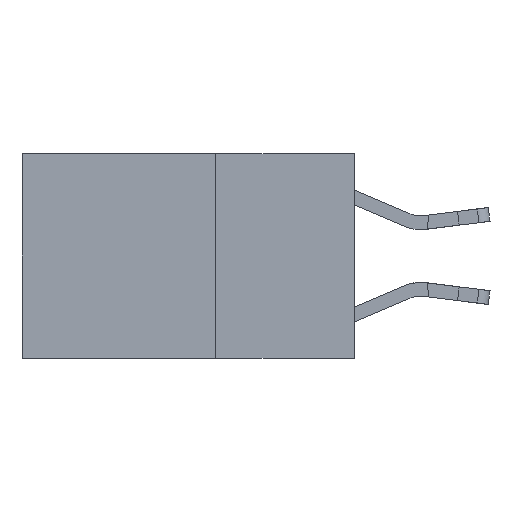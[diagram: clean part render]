
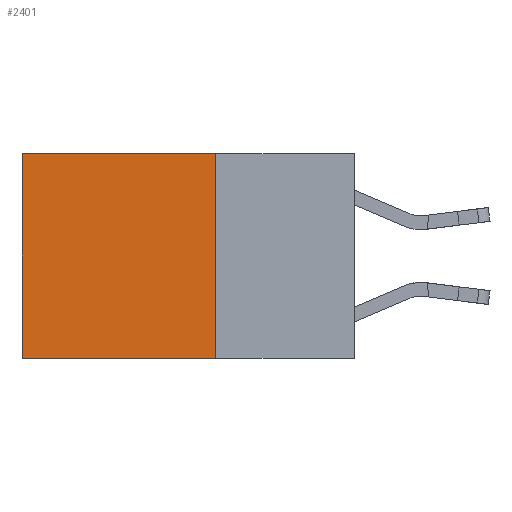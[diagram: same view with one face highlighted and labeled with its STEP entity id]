
A CAD part, left-side view. The second image highlights one B-rep face of the part: STEP entity #2401.
In plain terms, the highlighted planar face has unit normal (-1, 0, 0).
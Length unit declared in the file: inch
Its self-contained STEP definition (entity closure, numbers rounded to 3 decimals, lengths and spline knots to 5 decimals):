
#825 = DIRECTION ( 'NONE',  ( 1., 0., 0. ) ) ;
#909 = VECTOR ( 'NONE', #12028, 39.37008 ) ;
#1148 = VECTOR ( 'NONE', #17235, 39.37008 ) ;
#1781 = CARTESIAN_POINT ( 'NONE',  ( 0.2625, 0.25, -0.37 ) ) ;
#2177 = AXIS2_PLACEMENT_3D ( 'NONE', #2512, #825, #15468 ) ;
#2401 = ADVANCED_FACE ( 'NONE', ( #4428 ), #19159, .F. ) ;
#2512 = CARTESIAN_POINT ( 'NONE',  ( 0.2625, 0.25, 0. ) ) ;
#3327 = CARTESIAN_POINT ( 'NONE',  ( 0.2625, 0.25, 0. ) ) ;
#3854 = CARTESIAN_POINT ( 'NONE',  ( 0.2625, 0.6, 0. ) ) ;
#4428 = FACE_OUTER_BOUND ( 'NONE', #4574, .T. ) ;
#4574 = EDGE_LOOP ( 'NONE', ( #14198, #22032, #8358, #16067 ) ) ;
#7031 = CARTESIAN_POINT ( 'NONE',  ( 0.2625, 0.25, 0. ) ) ;
#7167 = DIRECTION ( 'NONE',  ( 0., 1., 0. ) ) ;
#8117 = DIRECTION ( 'NONE',  ( 0., 0., -1. ) ) ;
#8358 = ORIENTED_EDGE ( 'NONE', *, *, #12538, .F. ) ;
#8605 = CARTESIAN_POINT ( 'NONE',  ( 0.2625, 0.6, 0. ) ) ;
#9194 = EDGE_CURVE ( 'NONE', #16726, #17531, #23234, .T. ) ;
#12028 = DIRECTION ( 'NONE',  ( 0., 0., -1. ) ) ;
#12380 = VECTOR ( 'NONE', #7167, 39.37008 ) ;
#12538 = EDGE_CURVE ( 'NONE', #16726, #15428, #17243, .T. ) ;
#13546 = CARTESIAN_POINT ( 'NONE',  ( 0.2625, 0.25, 0. ) ) ;
#14166 = LINE ( 'NONE', #8605, #909 ) ;
#14198 = ORIENTED_EDGE ( 'NONE', *, *, #19023, .T. ) ;
#14261 = LINE ( 'NONE', #1781, #12380 ) ;
#15428 = VERTEX_POINT ( 'NONE', #23345 ) ;
#15468 = DIRECTION ( 'NONE',  ( 0., 0., -1. ) ) ;
#16067 = ORIENTED_EDGE ( 'NONE', *, *, #9194, .T. ) ;
#16726 = VERTEX_POINT ( 'NONE', #7031 ) ;
#16929 = CARTESIAN_POINT ( 'NONE',  ( 0.2625, 0.6, -0.37 ) ) ;
#17235 = DIRECTION ( 'NONE',  ( 0., 1., 0. ) ) ;
#17243 = LINE ( 'NONE', #13546, #22647 ) ;
#17531 = VERTEX_POINT ( 'NONE', #3854 ) ;
#18919 = VERTEX_POINT ( 'NONE', #16929 ) ;
#19023 = EDGE_CURVE ( 'NONE', #17531, #18919, #14166, .T. ) ;
#19159 = PLANE ( 'NONE',  #2177 ) ;
#21137 = EDGE_CURVE ( 'NONE', #15428, #18919, #14261, .T. ) ;
#22032 = ORIENTED_EDGE ( 'NONE', *, *, #21137, .F. ) ;
#22647 = VECTOR ( 'NONE', #8117, 39.37008 ) ;
#23234 = LINE ( 'NONE', #3327, #1148 ) ;
#23345 = CARTESIAN_POINT ( 'NONE',  ( 0.2625, 0.25, -0.37 ) ) ;
